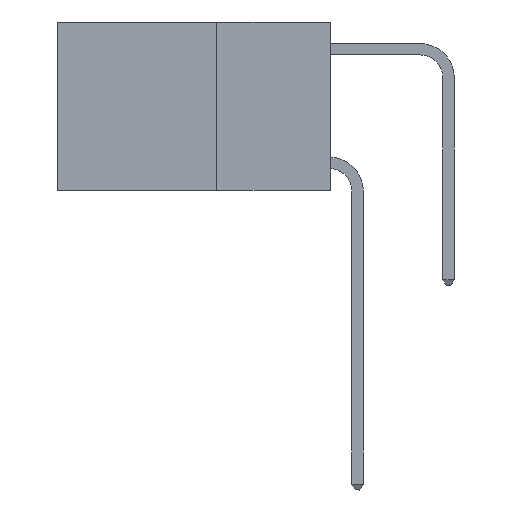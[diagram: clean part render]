
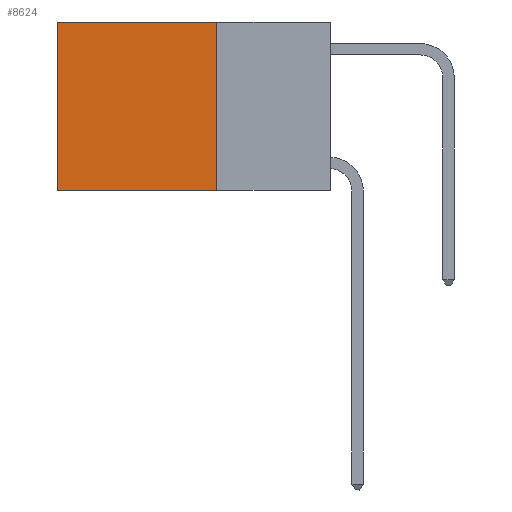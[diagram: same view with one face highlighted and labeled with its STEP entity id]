
A CAD part, left-side view. The second image highlights one B-rep face of the part: STEP entity #8624.
In plain terms, the highlighted planar face has unit normal (-1, 0, 0).
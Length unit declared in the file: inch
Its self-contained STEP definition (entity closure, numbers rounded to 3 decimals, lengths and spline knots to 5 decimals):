
#1365 = CARTESIAN_POINT ( 'NONE',  ( 0.2625, 0.25, 0. ) ) ;
#2984 = ORIENTED_EDGE ( 'NONE', *, *, #17871, .T. ) ;
#3624 = CARTESIAN_POINT ( 'NONE',  ( 0.2625, 0.25, 0. ) ) ;
#3779 = VERTEX_POINT ( 'NONE', #3817 ) ;
#3817 = CARTESIAN_POINT ( 'NONE',  ( 0.2625, 0.6, 0. ) ) ;
#4535 = ORIENTED_EDGE ( 'NONE', *, *, #14682, .F. ) ;
#5707 = LINE ( 'NONE', #3624, #23931 ) ;
#6117 = DIRECTION ( 'NONE',  ( 0., 0., -1. ) ) ;
#6654 = FACE_OUTER_BOUND ( 'NONE', #21107, .T. ) ;
#6780 = VECTOR ( 'NONE', #20570, 39.37008 ) ;
#6988 = LINE ( 'NONE', #29191, #13551 ) ;
#8624 = ADVANCED_FACE ( 'NONE', ( #6654 ), #18708, .F. ) ;
#9638 = VERTEX_POINT ( 'NONE', #14746 ) ;
#10590 = VERTEX_POINT ( 'NONE', #11417 ) ;
#10739 = CARTESIAN_POINT ( 'NONE',  ( 0.2625, 0.6, -0.37 ) ) ;
#11417 = CARTESIAN_POINT ( 'NONE',  ( 0.2625, 0.25, -0.37 ) ) ;
#13330 = LINE ( 'NONE', #15546, #6780 ) ;
#13551 = VECTOR ( 'NONE', #14418, 39.37008 ) ;
#13797 = DIRECTION ( 'NONE',  ( 0., 0., -1. ) ) ;
#14418 = DIRECTION ( 'NONE',  ( 0., 1., 0. ) ) ;
#14682 = EDGE_CURVE ( 'NONE', #10590, #16431, #6988, .T. ) ;
#14746 = CARTESIAN_POINT ( 'NONE',  ( 0.2625, 0.25, 0. ) ) ;
#15546 = CARTESIAN_POINT ( 'NONE',  ( 0.2625, 0.25, 0. ) ) ;
#16431 = VERTEX_POINT ( 'NONE', #10739 ) ;
#17871 = EDGE_CURVE ( 'NONE', #9638, #3779, #13330, .T. ) ;
#18231 = DIRECTION ( 'NONE',  ( 0., 0., -1. ) ) ;
#18575 = VECTOR ( 'NONE', #18231, 39.37008 ) ;
#18708 = PLANE ( 'NONE',  #31384 ) ;
#20570 = DIRECTION ( 'NONE',  ( 0., 1., 0. ) ) ;
#21107 = EDGE_LOOP ( 'NONE', ( #29100, #4535, #28145, #2984 ) ) ;
#22412 = EDGE_CURVE ( 'NONE', #3779, #16431, #30884, .T. ) ;
#23111 = CARTESIAN_POINT ( 'NONE',  ( 0.2625, 0.6, 0. ) ) ;
#23931 = VECTOR ( 'NONE', #6117, 39.37008 ) ;
#28145 = ORIENTED_EDGE ( 'NONE', *, *, #29784, .F. ) ;
#28601 = DIRECTION ( 'NONE',  ( 1., 0., 0. ) ) ;
#29100 = ORIENTED_EDGE ( 'NONE', *, *, #22412, .T. ) ;
#29191 = CARTESIAN_POINT ( 'NONE',  ( 0.2625, 0.25, -0.37 ) ) ;
#29784 = EDGE_CURVE ( 'NONE', #9638, #10590, #5707, .T. ) ;
#30884 = LINE ( 'NONE', #23111, #18575 ) ;
#31384 = AXIS2_PLACEMENT_3D ( 'NONE', #1365, #28601, #13797 ) ;
